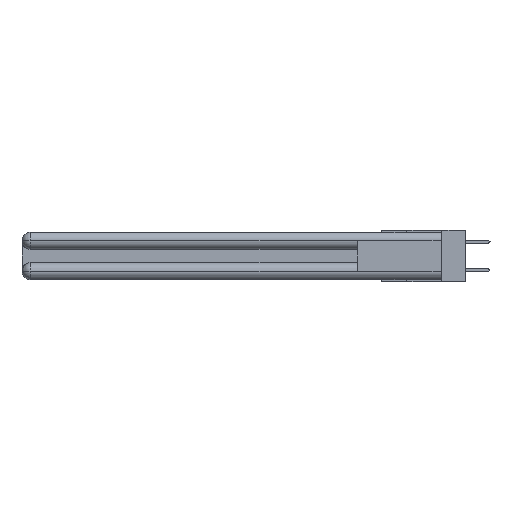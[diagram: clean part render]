
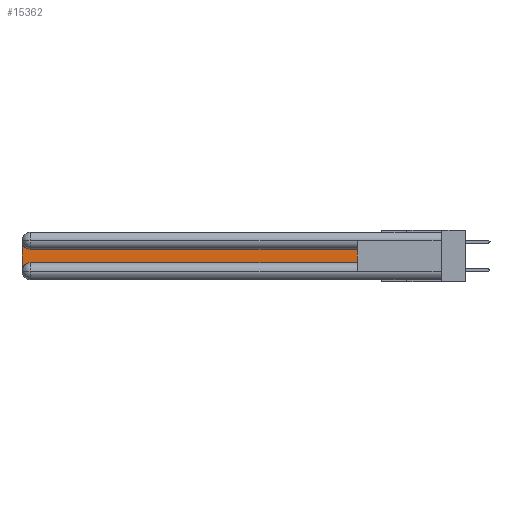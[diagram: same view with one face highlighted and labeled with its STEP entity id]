
A CAD part, left-side view. The second image highlights one B-rep face of the part: STEP entity #15362.
In plain terms, the highlighted planar face has unit normal (-1, 0, 0).
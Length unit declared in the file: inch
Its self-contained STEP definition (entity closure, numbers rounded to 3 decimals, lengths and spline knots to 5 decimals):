
#171 = VERTEX_POINT ( 'NONE', #2233 ) ;
#376 = DIRECTION ( 'NONE',  ( 1., 0., 0. ) ) ;
#1440 = EDGE_CURVE ( 'NONE', #1540, #13812, #14585, .T. ) ;
#1540 = VERTEX_POINT ( 'NONE', #2494 ) ;
#2054 = LINE ( 'NONE', #24727, #6110 ) ;
#2233 = CARTESIAN_POINT ( 'NONE',  ( 0.075, 2.94, -0.1225 ) ) ;
#2494 = CARTESIAN_POINT ( 'NONE',  ( 0.075, 2.94, -0.2175 ) ) ;
#2939 = ORIENTED_EDGE ( 'NONE', *, *, #8105, .T. ) ;
#3089 = DIRECTION ( 'NONE',  ( 0., 0., 1. ) ) ;
#4454 = FACE_OUTER_BOUND ( 'NONE', #21640, .T. ) ;
#5577 = LINE ( 'NONE', #16822, #22775 ) ;
#5788 = EDGE_CURVE ( 'NONE', #13855, #11734, #2054, .T. ) ;
#6110 = VECTOR ( 'NONE', #13012, 39.37008 ) ;
#7187 = CARTESIAN_POINT ( 'NONE',  ( 0.075, 0.6, -0.2175 ) ) ;
#8105 = EDGE_CURVE ( 'NONE', #171, #13855, #11883, .T. ) ;
#8196 = AXIS2_PLACEMENT_3D ( 'NONE', #29637, #29734, #24889 ) ;
#10701 = ORIENTED_EDGE ( 'NONE', *, *, #1440, .T. ) ;
#10924 = DIRECTION ( 'NONE',  ( 0., -1., 0. ) ) ;
#11069 = ORIENTED_EDGE ( 'NONE', *, *, #23991, .T. ) ;
#11339 = EDGE_CURVE ( 'NONE', #13812, #27242, #18195, .T. ) ;
#11734 = VERTEX_POINT ( 'NONE', #17168 ) ;
#11883 = CIRCLE ( 'NONE', #26076, 0.06 ) ;
#12108 = CARTESIAN_POINT ( 'NONE',  ( 0.075, 2.94, -0.0625 ) ) ;
#12244 = DIRECTION ( 'NONE',  ( 0., 1., 0. ) ) ;
#13012 = DIRECTION ( 'NONE',  ( 0., 0., -1. ) ) ;
#13388 = ORIENTED_EDGE ( 'NONE', *, *, #21866, .T. ) ;
#13812 = VERTEX_POINT ( 'NONE', #22729 ) ;
#13826 = VECTOR ( 'NONE', #3089, 39.37008 ) ;
#13855 = VERTEX_POINT ( 'NONE', #17910 ) ;
#14210 = CARTESIAN_POINT ( 'NONE',  ( 0.075, 2.94, -0.2775 ) ) ;
#14385 = AXIS2_PLACEMENT_3D ( 'NONE', #14210, #21040, #16133 ) ;
#14585 = LINE ( 'NONE', #26824, #18189 ) ;
#15021 = ORIENTED_EDGE ( 'NONE', *, *, #5788, .T. ) ;
#15362 = ADVANCED_FACE ( 'NONE', ( #4454 ), #24702, .F. ) ;
#16133 = DIRECTION ( 'NONE',  ( 0., 0., -1. ) ) ;
#16822 = CARTESIAN_POINT ( 'NONE',  ( 0.075, 0.6, -0.1225 ) ) ;
#16985 = DIRECTION ( 'NONE',  ( 0., 0., -1. ) ) ;
#17168 = CARTESIAN_POINT ( 'NONE',  ( 0.075, 3., -0.2775 ) ) ;
#17910 = CARTESIAN_POINT ( 'NONE',  ( 0.075, 3., -0.0625 ) ) ;
#18189 = VECTOR ( 'NONE', #10924, 39.37008 ) ;
#18195 = LINE ( 'NONE', #7187, #13826 ) ;
#19788 = ORIENTED_EDGE ( 'NONE', *, *, #11339, .T. ) ;
#21040 = DIRECTION ( 'NONE',  ( 1., 0., 0. ) ) ;
#21640 = EDGE_LOOP ( 'NONE', ( #11069, #2939, #15021, #13388, #10701, #19788 ) ) ;
#21866 = EDGE_CURVE ( 'NONE', #11734, #1540, #24336, .T. ) ;
#22729 = CARTESIAN_POINT ( 'NONE',  ( 0.075, 0.6, -0.2175 ) ) ;
#22775 = VECTOR ( 'NONE', #12244, 39.37008 ) ;
#23991 = EDGE_CURVE ( 'NONE', #27242, #171, #5577, .T. ) ;
#24336 = CIRCLE ( 'NONE', #14385, 0.06 ) ;
#24702 = PLANE ( 'NONE',  #8196 ) ;
#24727 = CARTESIAN_POINT ( 'NONE',  ( 0.075, 3., -0.2175 ) ) ;
#24889 = DIRECTION ( 'NONE',  ( 0., 0., -1. ) ) ;
#25645 = CARTESIAN_POINT ( 'NONE',  ( 0.075, 0.6, -0.1225 ) ) ;
#26076 = AXIS2_PLACEMENT_3D ( 'NONE', #12108, #376, #16985 ) ;
#26824 = CARTESIAN_POINT ( 'NONE',  ( 0.075, 0.6, -0.2175 ) ) ;
#27242 = VERTEX_POINT ( 'NONE', #25645 ) ;
#29637 = CARTESIAN_POINT ( 'NONE',  ( 0.075, 3., -0.1225 ) ) ;
#29734 = DIRECTION ( 'NONE',  ( 1., 0., 0. ) ) ;
